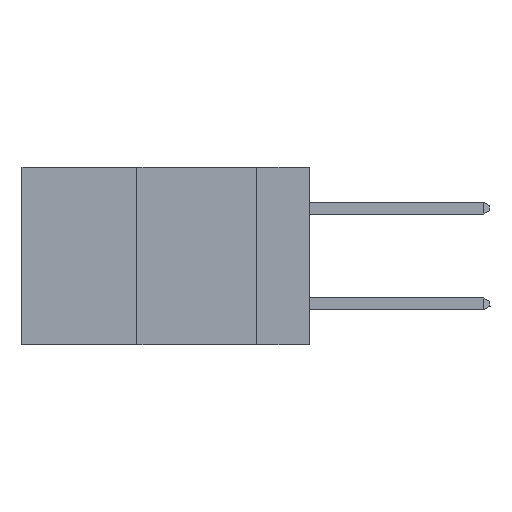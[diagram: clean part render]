
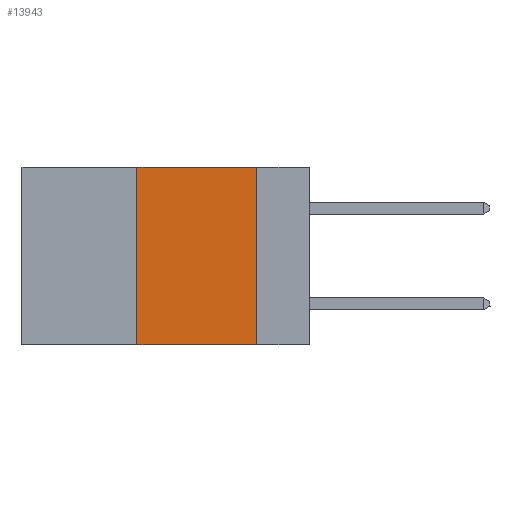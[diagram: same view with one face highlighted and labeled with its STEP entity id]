
A CAD part, left-side view. The second image highlights one B-rep face of the part: STEP entity #13943.
In plain terms, the highlighted planar face has unit normal (-1, 0, 0).
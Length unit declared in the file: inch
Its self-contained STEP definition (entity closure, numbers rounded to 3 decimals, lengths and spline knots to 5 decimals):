
#201 = DIRECTION ( 'NONE',  ( 0., -1., 0. ) ) ;
#788 = CARTESIAN_POINT ( 'NONE',  ( 0., 0.6, 0. ) ) ;
#800 = ORIENTED_EDGE ( 'NONE', *, *, #8743, .F. ) ;
#1952 = CARTESIAN_POINT ( 'NONE',  ( 0., 0.6, 0. ) ) ;
#2158 = DIRECTION ( 'NONE',  ( 0., 0., -1. ) ) ;
#2159 = LINE ( 'NONE', #14433, #10241 ) ;
#2267 = CARTESIAN_POINT ( 'NONE',  ( 0., 0.36, 0. ) ) ;
#2351 = VECTOR ( 'NONE', #201, 39.37008 ) ;
#2834 = DIRECTION ( 'NONE',  ( 0., 0., -1. ) ) ;
#3345 = LINE ( 'NONE', #1952, #2351 ) ;
#3547 = EDGE_LOOP ( 'NONE', ( #800, #9731, #7247, #16022 ) ) ;
#3643 = VERTEX_POINT ( 'NONE', #14833 ) ;
#3984 = LINE ( 'NONE', #9947, #14017 ) ;
#4018 = EDGE_CURVE ( 'NONE', #11003, #4381, #2159, .T. ) ;
#4381 = VERTEX_POINT ( 'NONE', #18497 ) ;
#5906 = CARTESIAN_POINT ( 'NONE',  ( 0., 0.36, -0.37 ) ) ;
#5924 = EDGE_CURVE ( 'NONE', #11003, #15535, #3984, .T. ) ;
#7247 = ORIENTED_EDGE ( 'NONE', *, *, #5924, .F. ) ;
#8015 = DIRECTION ( 'NONE',  ( 1., 0., 0. ) ) ;
#8469 = DIRECTION ( 'NONE',  ( 0., 0., 1. ) ) ;
#8743 = EDGE_CURVE ( 'NONE', #3643, #4381, #12888, .T. ) ;
#9731 = ORIENTED_EDGE ( 'NONE', *, *, #17164, .F. ) ;
#9947 = CARTESIAN_POINT ( 'NONE',  ( 0., 0.36, 0. ) ) ;
#10010 = VECTOR ( 'NONE', #2834, 39.37008 ) ;
#10241 = VECTOR ( 'NONE', #17723, 39.37008 ) ;
#11003 = VERTEX_POINT ( 'NONE', #5906 ) ;
#12034 = AXIS2_PLACEMENT_3D ( 'NONE', #788, #8015, #2158 ) ;
#12405 = FACE_OUTER_BOUND ( 'NONE', #3547, .T. ) ;
#12791 = PLANE ( 'NONE',  #12034 ) ;
#12888 = LINE ( 'NONE', #19091, #10010 ) ;
#13943 = ADVANCED_FACE ( 'NONE', ( #12405 ), #12791, .F. ) ;
#14017 = VECTOR ( 'NONE', #8469, 39.37008 ) ;
#14433 = CARTESIAN_POINT ( 'NONE',  ( 0., 0.6, -0.37 ) ) ;
#14833 = CARTESIAN_POINT ( 'NONE',  ( 0., 0.11, 0. ) ) ;
#15535 = VERTEX_POINT ( 'NONE', #2267 ) ;
#16022 = ORIENTED_EDGE ( 'NONE', *, *, #4018, .T. ) ;
#17164 = EDGE_CURVE ( 'NONE', #15535, #3643, #3345, .T. ) ;
#17723 = DIRECTION ( 'NONE',  ( 0., -1., 0. ) ) ;
#18497 = CARTESIAN_POINT ( 'NONE',  ( 0., 0.11, -0.37 ) ) ;
#19091 = CARTESIAN_POINT ( 'NONE',  ( 0., 0.11, 0. ) ) ;
